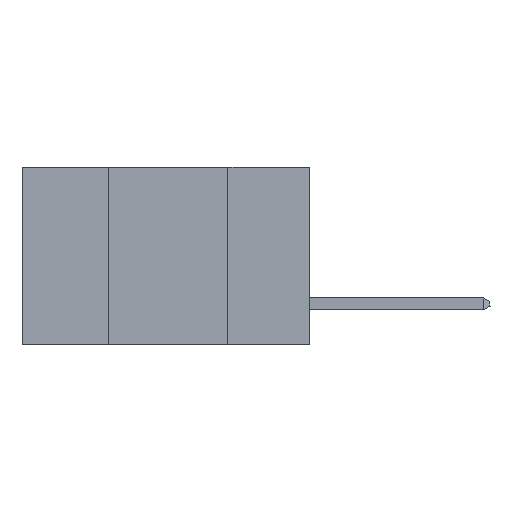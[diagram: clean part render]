
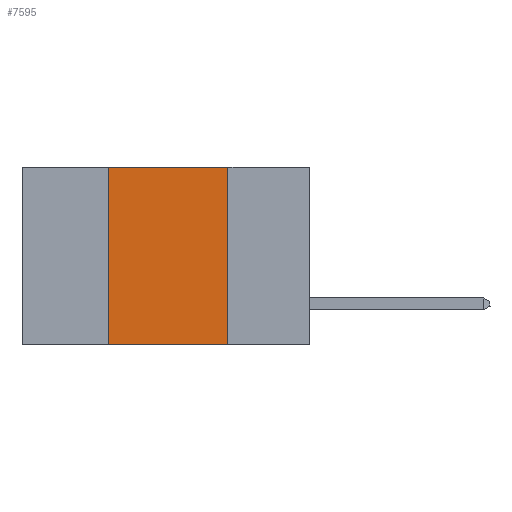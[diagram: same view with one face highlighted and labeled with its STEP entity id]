
A CAD part, left-side view. The second image highlights one B-rep face of the part: STEP entity #7595.
In plain terms, the highlighted planar face has unit normal (-1, 0, 0).
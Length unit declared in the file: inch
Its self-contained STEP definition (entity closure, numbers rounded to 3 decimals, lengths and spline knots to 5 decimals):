
#2085 = VERTEX_POINT ( 'NONE', #30325 ) ;
#4349 = DIRECTION ( 'NONE',  ( 0., 0., 1. ) ) ;
#4605 = ORIENTED_EDGE ( 'NONE', *, *, #7045, .T. ) ;
#4941 = PLANE ( 'NONE',  #19321 ) ;
#6785 = EDGE_LOOP ( 'NONE', ( #9127, #29762, #23840, #4605 ) ) ;
#7045 = EDGE_CURVE ( 'NONE', #46495, #21635, #34551, .T. ) ;
#7595 = ADVANCED_FACE ( 'NONE', ( #22196 ), #4941, .F. ) ;
#8189 = CARTESIAN_POINT ( 'NONE',  ( 0., 0.17, 0. ) ) ;
#8451 = VECTOR ( 'NONE', #16058, 39.37008 ) ;
#9127 = ORIENTED_EDGE ( 'NONE', *, *, #35802, .F. ) ;
#11550 = CARTESIAN_POINT ( 'NONE',  ( 0., 0.42, 0. ) ) ;
#11827 = CARTESIAN_POINT ( 'NONE',  ( 0., 0.17, -0.37 ) ) ;
#11969 = DIRECTION ( 'NONE',  ( 1., 0., 0. ) ) ;
#14826 = EDGE_CURVE ( 'NONE', #46495, #2085, #39731, .T. ) ;
#15268 = VECTOR ( 'NONE', #27483, 39.37008 ) ;
#16058 = DIRECTION ( 'NONE',  ( 0., -1., 0. ) ) ;
#16363 = DIRECTION ( 'NONE',  ( 0., 0., -1. ) ) ;
#19321 = AXIS2_PLACEMENT_3D ( 'NONE', #23535, #11969, #16363 ) ;
#19936 = CARTESIAN_POINT ( 'NONE',  ( 0., 0.6, 0. ) ) ;
#21635 = VERTEX_POINT ( 'NONE', #11827 ) ;
#22196 = FACE_OUTER_BOUND ( 'NONE', #6785, .T. ) ;
#23535 = CARTESIAN_POINT ( 'NONE',  ( 0., 0.6, 0. ) ) ;
#23840 = ORIENTED_EDGE ( 'NONE', *, *, #14826, .F. ) ;
#27483 = DIRECTION ( 'NONE',  ( 0., -1., 0. ) ) ;
#27703 = VECTOR ( 'NONE', #29049, 39.37008 ) ;
#28339 = EDGE_CURVE ( 'NONE', #2085, #32652, #33467, .T. ) ;
#28935 = CARTESIAN_POINT ( 'NONE',  ( 0., 0.42, -0.37 ) ) ;
#29049 = DIRECTION ( 'NONE',  ( 0., 0., -1. ) ) ;
#29762 = ORIENTED_EDGE ( 'NONE', *, *, #28339, .F. ) ;
#29824 = VECTOR ( 'NONE', #4349, 39.37008 ) ;
#30325 = CARTESIAN_POINT ( 'NONE',  ( 0., 0.42, 0. ) ) ;
#31779 = LINE ( 'NONE', #40480, #27703 ) ;
#32652 = VERTEX_POINT ( 'NONE', #8189 ) ;
#33467 = LINE ( 'NONE', #19936, #8451 ) ;
#34551 = LINE ( 'NONE', #42852, #15268 ) ;
#35802 = EDGE_CURVE ( 'NONE', #32652, #21635, #31779, .T. ) ;
#39731 = LINE ( 'NONE', #11550, #29824 ) ;
#40480 = CARTESIAN_POINT ( 'NONE',  ( 0., 0.17, 0. ) ) ;
#42852 = CARTESIAN_POINT ( 'NONE',  ( 0., 0.6, -0.37 ) ) ;
#46495 = VERTEX_POINT ( 'NONE', #28935 ) ;
